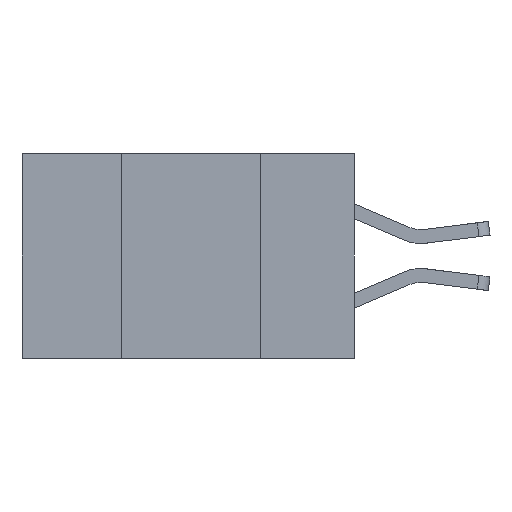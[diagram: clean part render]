
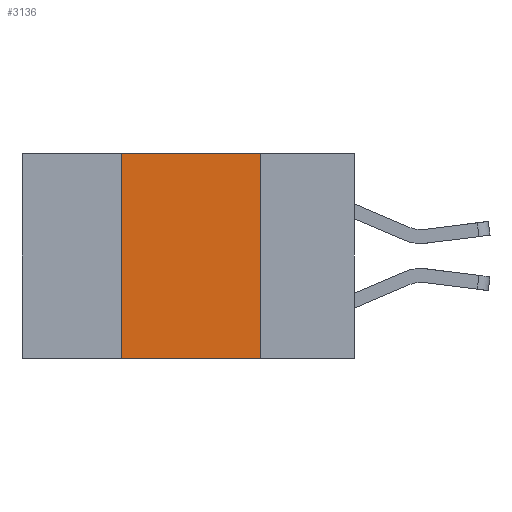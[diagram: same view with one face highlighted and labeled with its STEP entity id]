
A CAD part, left-side view. The second image highlights one B-rep face of the part: STEP entity #3136.
In plain terms, the highlighted planar face has unit normal (-1, 0, 0).
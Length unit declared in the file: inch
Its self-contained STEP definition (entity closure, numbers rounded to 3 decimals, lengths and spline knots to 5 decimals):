
#312 = PLANE ( 'NONE',  #7918 ) ;
#480 = CARTESIAN_POINT ( 'NONE',  ( 0., 0.6, 0. ) ) ;
#687 = DIRECTION ( 'NONE',  ( 0., -1., 0. ) ) ;
#803 = VERTEX_POINT ( 'NONE', #3492 ) ;
#1613 = LINE ( 'NONE', #2331, #7443 ) ;
#1800 = ORIENTED_EDGE ( 'NONE', *, *, #4703, .T. ) ;
#2331 = CARTESIAN_POINT ( 'NONE',  ( 0., 0.6, -0.37 ) ) ;
#2474 = CARTESIAN_POINT ( 'NONE',  ( 0., 0.42, -0.37 ) ) ;
#3136 = ADVANCED_FACE ( 'NONE', ( #3792 ), #312, .F. ) ;
#3191 = VECTOR ( 'NONE', #3261, 39.37008 ) ;
#3217 = DIRECTION ( 'NONE',  ( 0., 0., 1. ) ) ;
#3261 = DIRECTION ( 'NONE',  ( 0., -1., 0. ) ) ;
#3492 = CARTESIAN_POINT ( 'NONE',  ( 0., 0.17, -0.37 ) ) ;
#3792 = FACE_OUTER_BOUND ( 'NONE', #7802, .T. ) ;
#4081 = CARTESIAN_POINT ( 'NONE',  ( 0., 0.6, 0. ) ) ;
#4438 = DIRECTION ( 'NONE',  ( 0., 0., -1. ) ) ;
#4703 = EDGE_CURVE ( 'NONE', #5257, #803, #1613, .T. ) ;
#5045 = ORIENTED_EDGE ( 'NONE', *, *, #8799, .F. ) ;
#5232 = CARTESIAN_POINT ( 'NONE',  ( 0., 0.42, 0. ) ) ;
#5257 = VERTEX_POINT ( 'NONE', #5564 ) ;
#5307 = VERTEX_POINT ( 'NONE', #5232 ) ;
#5564 = CARTESIAN_POINT ( 'NONE',  ( 0., 0.42, -0.37 ) ) ;
#5939 = VERTEX_POINT ( 'NONE', #10296 ) ;
#6295 = VECTOR ( 'NONE', #3217, 39.37008 ) ;
#7099 = DIRECTION ( 'NONE',  ( 0., 0., -1. ) ) ;
#7443 = VECTOR ( 'NONE', #687, 39.37008 ) ;
#7655 = EDGE_CURVE ( 'NONE', #5939, #803, #10339, .T. ) ;
#7802 = EDGE_LOOP ( 'NONE', ( #10643, #7949, #5045, #1800 ) ) ;
#7918 = AXIS2_PLACEMENT_3D ( 'NONE', #480, #10346, #7099 ) ;
#7949 = ORIENTED_EDGE ( 'NONE', *, *, #9312, .F. ) ;
#8132 = LINE ( 'NONE', #2474, #6295 ) ;
#8668 = VECTOR ( 'NONE', #4438, 39.37008 ) ;
#8799 = EDGE_CURVE ( 'NONE', #5257, #5307, #8132, .T. ) ;
#8995 = LINE ( 'NONE', #4081, #3191 ) ;
#9312 = EDGE_CURVE ( 'NONE', #5307, #5939, #8995, .T. ) ;
#10178 = CARTESIAN_POINT ( 'NONE',  ( 0., 0.17, -0.37 ) ) ;
#10296 = CARTESIAN_POINT ( 'NONE',  ( 0., 0.17, 0. ) ) ;
#10339 = LINE ( 'NONE', #10178, #8668 ) ;
#10346 = DIRECTION ( 'NONE',  ( 1., 0., 0. ) ) ;
#10643 = ORIENTED_EDGE ( 'NONE', *, *, #7655, .F. ) ;
